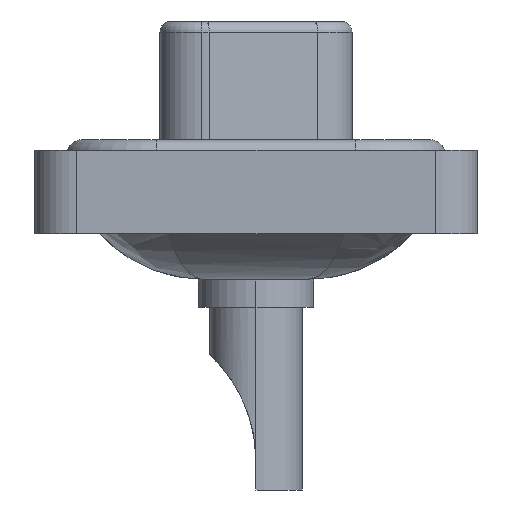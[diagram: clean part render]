
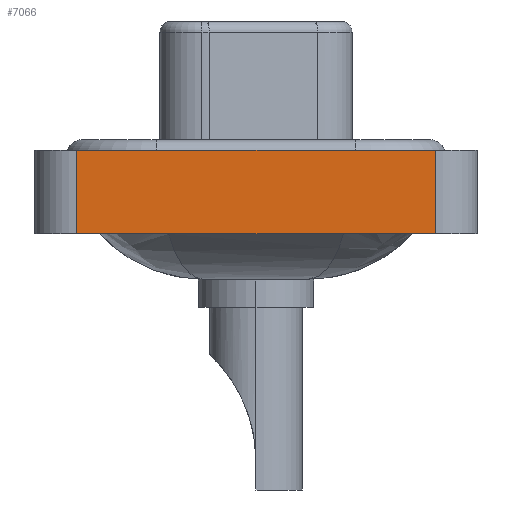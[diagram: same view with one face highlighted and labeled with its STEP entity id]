
A CAD part, left-side view. The second image highlights one B-rep face of the part: STEP entity #7066.
In plain terms, the highlighted planar face has unit normal (-1, 0, 0).
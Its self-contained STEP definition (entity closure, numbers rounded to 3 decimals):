
#323 = LINE ( 'NONE', #12029, #4131 ) ;
#2060 = LINE ( 'NONE', #10380, #10891 ) ;
#2225 = VECTOR ( 'NONE', #13150, 1000. ) ;
#3229 = CARTESIAN_POINT ( 'NONE',  ( -7.35, 8.55, 0.4 ) ) ;
#3793 = DIRECTION ( 'NONE',  ( 0., 0., 1. ) ) ;
#4131 = VECTOR ( 'NONE', #3793, 1000. ) ;
#4838 = CARTESIAN_POINT ( 'NONE',  ( -7.35, 8.55, -3.6 ) ) ;
#5183 = ORIENTED_EDGE ( 'NONE', *, *, #8205, .F. ) ;
#6151 = EDGE_CURVE ( 'NONE', #13065, #17101, #22164, .T. ) ;
#7066 = ADVANCED_FACE ( 'NONE', ( #10170 ), #20167, .T. ) ;
#8205 = EDGE_CURVE ( 'NONE', #11249, #13065, #323, .T. ) ;
#8687 = VECTOR ( 'NONE', #17026, 1000. ) ;
#10059 = DIRECTION ( 'NONE',  ( -1., 0., 0. ) ) ;
#10170 = FACE_OUTER_BOUND ( 'NONE', #16252, .T. ) ;
#10380 = CARTESIAN_POINT ( 'NONE',  ( -7.35, -8.55, -3.6 ) ) ;
#10891 = VECTOR ( 'NONE', #20815, 1000. ) ;
#11249 = VERTEX_POINT ( 'NONE', #4838 ) ;
#11863 = CARTESIAN_POINT ( 'NONE',  ( -7.35, -8.55, 0.4 ) ) ;
#12029 = CARTESIAN_POINT ( 'NONE',  ( -7.35, 8.55, -3.6 ) ) ;
#13065 = VERTEX_POINT ( 'NONE', #3229 ) ;
#13150 = DIRECTION ( 'NONE',  ( 0., 0., 1. ) ) ;
#13453 = DIRECTION ( 'NONE',  ( 0., 0., 1. ) ) ;
#14139 = CARTESIAN_POINT ( 'NONE',  ( -7.35, -8.55, 0.4 ) ) ;
#14912 = ORIENTED_EDGE ( 'NONE', *, *, #16793, .T. ) ;
#16252 = EDGE_LOOP ( 'NONE', ( #17591, #16880, #5183, #14912 ) ) ;
#16793 = EDGE_CURVE ( 'NONE', #11249, #20545, #2060, .T. ) ;
#16880 = ORIENTED_EDGE ( 'NONE', *, *, #6151, .F. ) ;
#17026 = DIRECTION ( 'NONE',  ( 0., -1., 0. ) ) ;
#17101 = VERTEX_POINT ( 'NONE', #14139 ) ;
#17591 = ORIENTED_EDGE ( 'NONE', *, *, #18632, .T. ) ;
#18496 = CARTESIAN_POINT ( 'NONE',  ( -7.35, -8.55, -3.6 ) ) ;
#18631 = LINE ( 'NONE', #20311, #2225 ) ;
#18632 = EDGE_CURVE ( 'NONE', #20545, #17101, #18631, .T. ) ;
#20167 = PLANE ( 'NONE',  #22007 ) ;
#20311 = CARTESIAN_POINT ( 'NONE',  ( -7.35, -8.55, -3.6 ) ) ;
#20545 = VERTEX_POINT ( 'NONE', #21166 ) ;
#20815 = DIRECTION ( 'NONE',  ( 0., -1., 0. ) ) ;
#21166 = CARTESIAN_POINT ( 'NONE',  ( -7.35, -8.55, -3.6 ) ) ;
#22007 = AXIS2_PLACEMENT_3D ( 'NONE', #18496, #10059, #13453 ) ;
#22164 = LINE ( 'NONE', #11863, #8687 ) ;
